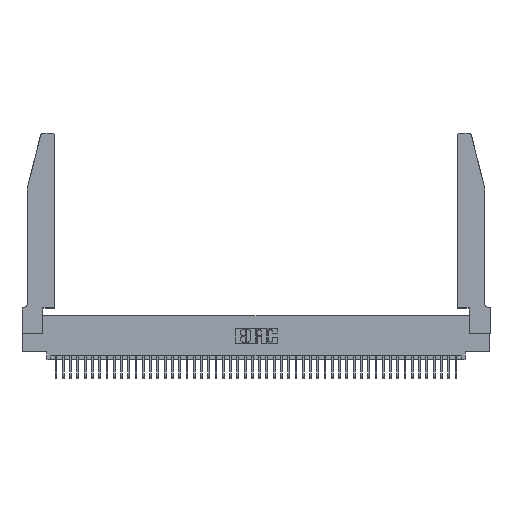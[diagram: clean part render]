
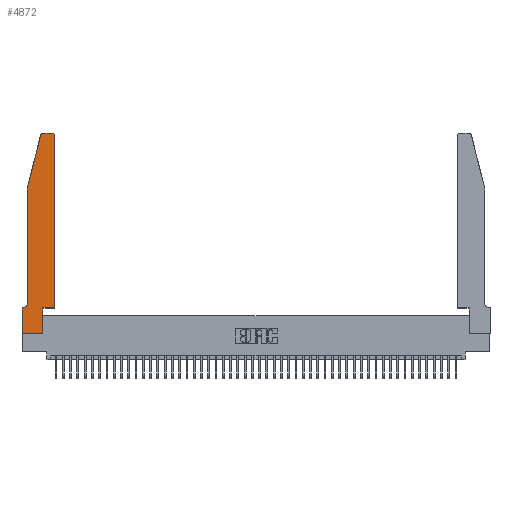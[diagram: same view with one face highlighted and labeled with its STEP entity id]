
A CAD part, top view. The second image highlights one B-rep face of the part: STEP entity #4872.
In plain terms, the highlighted planar face has unit normal (0, 0, 1).
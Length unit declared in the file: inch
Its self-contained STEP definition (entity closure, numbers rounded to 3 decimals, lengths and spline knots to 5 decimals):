
#2500 = CARTESIAN_POINT ( 'NONE',  ( 0.0055, 0.35, 0.37 ) ) ;
#3408 = LINE ( 'NONE', #34232, #42169 ) ;
#3600 = LINE ( 'NONE', #44549, #22579 ) ;
#3637 = DIRECTION ( 'NONE',  ( -1., 0., 0. ) ) ;
#3747 = VECTOR ( 'NONE', #16337, 39.37008 ) ;
#3781 = CARTESIAN_POINT ( 'NONE',  ( 0.4505, 2.72, 0.37 ) ) ;
#3951 = VERTEX_POINT ( 'NONE', #15344 ) ;
#4872 = ADVANCED_FACE ( 'NONE', ( #48018 ), #5404, .T. ) ;
#5404 = PLANE ( 'NONE',  #47804 ) ;
#6201 = LINE ( 'NONE', #8774, #3747 ) ;
#6711 = CARTESIAN_POINT ( 'NONE',  ( 0.284, 2.75, 0.37 ) ) ;
#7297 = EDGE_CURVE ( 'NONE', #39616, #8961, #40913, .T. ) ;
#7747 = ORIENTED_EDGE ( 'NONE', *, *, #22060, .T. ) ;
#7999 = AXIS2_PLACEMENT_3D ( 'NONE', #30494, #8016, #34218 ) ;
#8008 = ORIENTED_EDGE ( 'NONE', *, *, #47675, .T. ) ;
#8016 = DIRECTION ( 'NONE',  ( 0., 0., 1. ) ) ;
#8191 = EDGE_CURVE ( 'NONE', #29323, #39978, #12287, .T. ) ;
#8385 = VERTEX_POINT ( 'NONE', #48116 ) ;
#8774 = CARTESIAN_POINT ( 'NONE',  ( 0.0755, 2., 0.37 ) ) ;
#8961 = VERTEX_POINT ( 'NONE', #2500 ) ;
#8990 = VECTOR ( 'NONE', #32435, 39.37008 ) ;
#9315 = CARTESIAN_POINT ( 'NONE',  ( 0., 0.35, 0.37 ) ) ;
#11573 = ORIENTED_EDGE ( 'NONE', *, *, #25826, .T. ) ;
#12287 = LINE ( 'NONE', #28554, #30981 ) ;
#12573 = VERTEX_POINT ( 'NONE', #23040 ) ;
#12577 = LINE ( 'NONE', #32580, #8990 ) ;
#12647 = EDGE_CURVE ( 'NONE', #39978, #8385, #45985, .T. ) ;
#12671 = EDGE_CURVE ( 'NONE', #35421, #39616, #17468, .T. ) ;
#12696 = ORIENTED_EDGE ( 'NONE', *, *, #16483, .T. ) ;
#12721 = EDGE_CURVE ( 'NONE', #8385, #35421, #6201, .T. ) ;
#13033 = ORIENTED_EDGE ( 'NONE', *, *, #43324, .T. ) ;
#13129 = DIRECTION ( 'NONE',  ( 0., 0., 1. ) ) ;
#13284 = LINE ( 'NONE', #34016, #31991 ) ;
#13912 = EDGE_CURVE ( 'NONE', #3951, #12573, #13284, .T. ) ;
#14028 = AXIS2_PLACEMENT_3D ( 'NONE', #48525, #26322, #3637 ) ;
#14541 = VECTOR ( 'NONE', #44631, 39.37008 ) ;
#15344 = CARTESIAN_POINT ( 'NONE',  ( 0.2865, 0., 0.37 ) ) ;
#16024 = CARTESIAN_POINT ( 'NONE',  ( 0.284, 2.72, 0.37 ) ) ;
#16337 = DIRECTION ( 'NONE',  ( -0.239, -0.971, 0. ) ) ;
#16483 = EDGE_CURVE ( 'NONE', #20550, #3951, #48510, .T. ) ;
#17468 = LINE ( 'NONE', #45767, #44814 ) ;
#19739 = DIRECTION ( 'NONE',  ( 1., 0., 0. ) ) ;
#20348 = CARTESIAN_POINT ( 'NONE',  ( 0., 0., 0.37 ) ) ;
#20471 = ORIENTED_EDGE ( 'NONE', *, *, #13912, .T. ) ;
#20550 = VERTEX_POINT ( 'NONE', #38381 ) ;
#21490 = VERTEX_POINT ( 'NONE', #41523 ) ;
#22060 = EDGE_CURVE ( 'NONE', #12573, #21490, #3600, .T. ) ;
#22368 = CARTESIAN_POINT ( 'NONE',  ( 0.0755, 0.35, 0.37 ) ) ;
#22579 = VECTOR ( 'NONE', #48277, 39.37008 ) ;
#23040 = CARTESIAN_POINT ( 'NONE',  ( 0.2865, 0.35, 0.37 ) ) ;
#24133 = DIRECTION ( 'NONE',  ( 1., 0., 0. ) ) ;
#25826 = EDGE_CURVE ( 'NONE', #21490, #30410, #3408, .T. ) ;
#26322 = DIRECTION ( 'NONE',  ( 0., 0., -1. ) ) ;
#28469 = EDGE_LOOP ( 'NONE', ( #46602, #32181, #30579, #35991, #32683, #8008, #36143, #12696, #20471, #7747, #11573, #13033 ) ) ;
#28554 = CARTESIAN_POINT ( 'NONE',  ( 0.2605, 2.75, 0.37 ) ) ;
#28826 = VECTOR ( 'NONE', #24133, 39.37008 ) ;
#29323 = VERTEX_POINT ( 'NONE', #37467 ) ;
#30410 = VERTEX_POINT ( 'NONE', #3781 ) ;
#30494 = CARTESIAN_POINT ( 'NONE',  ( 0.4205, 2.72, 0.37 ) ) ;
#30504 = DIRECTION ( 'NONE',  ( 0., 1., 0. ) ) ;
#30579 = ORIENTED_EDGE ( 'NONE', *, *, #12721, .T. ) ;
#30981 = VECTOR ( 'NONE', #47002, 39.37008 ) ;
#31069 = CARTESIAN_POINT ( 'NONE',  ( 0.0755, 0.42, 0.37 ) ) ;
#31991 = VECTOR ( 'NONE', #37735, 39.37008 ) ;
#32181 = ORIENTED_EDGE ( 'NONE', *, *, #12647, .T. ) ;
#32435 = DIRECTION ( 'NONE',  ( 0., -1., 0. ) ) ;
#32580 = CARTESIAN_POINT ( 'NONE',  ( 0., 0., 0.37 ) ) ;
#32683 = ORIENTED_EDGE ( 'NONE', *, *, #7297, .T. ) ;
#32728 = EDGE_CURVE ( 'NONE', #40672, #20550, #12577, .T. ) ;
#34016 = CARTESIAN_POINT ( 'NONE',  ( 0.2865, 0.35, 0.37 ) ) ;
#34218 = DIRECTION ( 'NONE',  ( 1., 0., 0. ) ) ;
#34232 = CARTESIAN_POINT ( 'NONE',  ( 0.4505, 0.35, 0.37 ) ) ;
#34391 = LINE ( 'NONE', #22368, #14541 ) ;
#35421 = VERTEX_POINT ( 'NONE', #36970 ) ;
#35991 = ORIENTED_EDGE ( 'NONE', *, *, #12671, .T. ) ;
#36143 = ORIENTED_EDGE ( 'NONE', *, *, #32728, .T. ) ;
#36970 = CARTESIAN_POINT ( 'NONE',  ( 0.0755, 2., 0.37 ) ) ;
#37060 = CIRCLE ( 'NONE', #7999, 0.03 ) ;
#37467 = CARTESIAN_POINT ( 'NONE',  ( 0.4205, 2.75, 0.37 ) ) ;
#37735 = DIRECTION ( 'NONE',  ( 0., 1., 0. ) ) ;
#38381 = CARTESIAN_POINT ( 'NONE',  ( 0., 0., 0.37 ) ) ;
#39137 = AXIS2_PLACEMENT_3D ( 'NONE', #16024, #42049, #19739 ) ;
#39166 = DIRECTION ( 'NONE',  ( 1., 0., 0. ) ) ;
#39616 = VERTEX_POINT ( 'NONE', #31069 ) ;
#39978 = VERTEX_POINT ( 'NONE', #6711 ) ;
#40672 = VERTEX_POINT ( 'NONE', #43923 ) ;
#40913 = CIRCLE ( 'NONE', #14028, 0.07 ) ;
#41523 = CARTESIAN_POINT ( 'NONE',  ( 0.4505, 0.35, 0.37 ) ) ;
#42049 = DIRECTION ( 'NONE',  ( 0., 0., 1. ) ) ;
#42169 = VECTOR ( 'NONE', #30504, 39.37008 ) ;
#43324 = EDGE_CURVE ( 'NONE', #30410, #29323, #37060, .T. ) ;
#43923 = CARTESIAN_POINT ( 'NONE',  ( 0., 0.35, 0.37 ) ) ;
#44549 = CARTESIAN_POINT ( 'NONE',  ( 0.4505, 0.35, 0.37 ) ) ;
#44631 = DIRECTION ( 'NONE',  ( -1., 0., 0. ) ) ;
#44814 = VECTOR ( 'NONE', #45599, 39.37008 ) ;
#45599 = DIRECTION ( 'NONE',  ( 0., -1., 0. ) ) ;
#45767 = CARTESIAN_POINT ( 'NONE',  ( 0.0755, 2., 0.37 ) ) ;
#45985 = CIRCLE ( 'NONE', #39137, 0.03 ) ;
#46602 = ORIENTED_EDGE ( 'NONE', *, *, #8191, .T. ) ;
#47002 = DIRECTION ( 'NONE',  ( -1., 0., 0. ) ) ;
#47675 = EDGE_CURVE ( 'NONE', #8961, #40672, #34391, .T. ) ;
#47804 = AXIS2_PLACEMENT_3D ( 'NONE', #9315, #13129, #39166 ) ;
#48018 = FACE_OUTER_BOUND ( 'NONE', #28469, .T. ) ;
#48116 = CARTESIAN_POINT ( 'NONE',  ( 0.25487, 2.72718, 0.37 ) ) ;
#48277 = DIRECTION ( 'NONE',  ( 1., 0., 0. ) ) ;
#48510 = LINE ( 'NONE', #20348, #28826 ) ;
#48525 = CARTESIAN_POINT ( 'NONE',  ( 0.0055, 0.42, 0.37 ) ) ;
